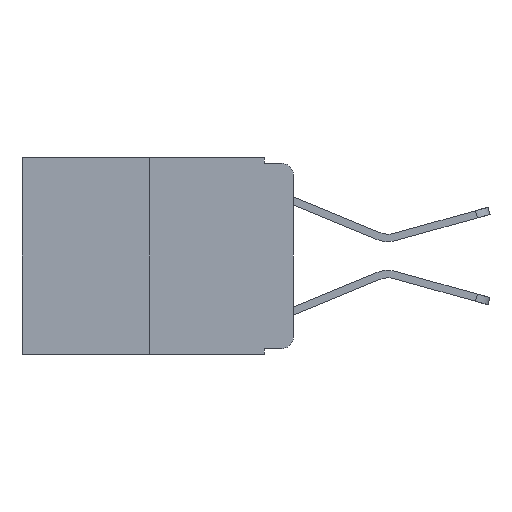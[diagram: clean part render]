
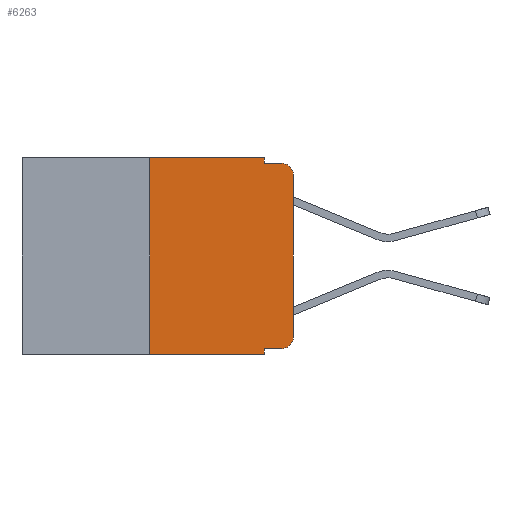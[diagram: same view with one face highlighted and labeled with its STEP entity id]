
A CAD part, left-side view. The second image highlights one B-rep face of the part: STEP entity #6263.
In plain terms, the highlighted planar face has unit normal (-1, 0, 0).
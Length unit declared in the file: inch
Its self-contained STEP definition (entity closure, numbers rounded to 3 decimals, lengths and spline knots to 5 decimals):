
#77 = VECTOR ( 'NONE', #7311, 39.37008 ) ;
#252 = VERTEX_POINT ( 'NONE', #10758 ) ;
#463 = LINE ( 'NONE', #9834, #77 ) ;
#479 = ORIENTED_EDGE ( 'NONE', *, *, #2550, .T. ) ;
#576 = CARTESIAN_POINT ( 'NONE',  ( 0., 0.051, -0.333 ) ) ;
#815 = VECTOR ( 'NONE', #9298, 39.37008 ) ;
#1189 = ORIENTED_EDGE ( 'NONE', *, *, #2565, .F. ) ;
#1667 = DIRECTION ( 'NONE',  ( 0., 0., -1. ) ) ;
#1753 = EDGE_CURVE ( 'NONE', #12235, #2693, #11513, .T. ) ;
#1758 = CARTESIAN_POINT ( 'NONE',  ( 0., 0.051, 0. ) ) ;
#2228 = EDGE_CURVE ( 'NONE', #6107, #11662, #3410, .T. ) ;
#2370 = CARTESIAN_POINT ( 'NONE',  ( 0., 0.02, -0.01 ) ) ;
#2532 = EDGE_CURVE ( 'NONE', #10820, #252, #11505, .T. ) ;
#2550 = EDGE_CURVE ( 'NONE', #252, #9981, #5945, .T. ) ;
#2552 = EDGE_CURVE ( 'NONE', #10318, #9981, #10676, .T. ) ;
#2565 = EDGE_CURVE ( 'NONE', #2693, #10318, #3234, .T. ) ;
#2580 = EDGE_CURVE ( 'NONE', #6107, #12235, #463, .T. ) ;
#2595 = EDGE_CURVE ( 'NONE', #3729, #11662, #2916, .T. ) ;
#2608 = EDGE_CURVE ( 'NONE', #3729, #10895, #10418, .T. ) ;
#2610 = EDGE_CURVE ( 'NONE', #10895, #10820, #5621, .T. ) ;
#2614 = VECTOR ( 'NONE', #9416, 39.37008 ) ;
#2693 = VERTEX_POINT ( 'NONE', #1758 ) ;
#2824 = CARTESIAN_POINT ( 'NONE',  ( 0., 0.25, -0.343 ) ) ;
#2873 = AXIS2_PLACEMENT_3D ( 'NONE', #7110, #12288, #1667 ) ;
#2916 = LINE ( 'NONE', #10233, #7987 ) ;
#3234 = LINE ( 'NONE', #4665, #815 ) ;
#3410 = LINE ( 'NONE', #9201, #10819 ) ;
#3729 = VERTEX_POINT ( 'NONE', #576 ) ;
#3899 = ORIENTED_EDGE ( 'NONE', *, *, #2580, .F. ) ;
#4074 = CARTESIAN_POINT ( 'NONE',  ( 0., 0., 0. ) ) ;
#4325 = DIRECTION ( 'NONE',  ( -1., 0., 0. ) ) ;
#4483 = DIRECTION ( 'NONE',  ( 0., 0., -1. ) ) ;
#4500 = CARTESIAN_POINT ( 'NONE',  ( 0., 0.02, -0.03 ) ) ;
#4665 = CARTESIAN_POINT ( 'NONE',  ( 0., 0.051, 0. ) ) ;
#5621 = CIRCLE ( 'NONE', #6164, 0.02 ) ;
#5795 = DIRECTION ( 'NONE',  ( 0., 0., -1. ) ) ;
#5832 = DIRECTION ( 'NONE',  ( -1., 0., 0. ) ) ;
#5945 = CIRCLE ( 'NONE', #10836, 0.02 ) ;
#5956 = ORIENTED_EDGE ( 'NONE', *, *, #2228, .T. ) ;
#6047 = CARTESIAN_POINT ( 'NONE',  ( 0., 0.051, -0.333 ) ) ;
#6105 = DIRECTION ( 'NONE',  ( 0., 0., 1. ) ) ;
#6107 = VERTEX_POINT ( 'NONE', #2824 ) ;
#6137 = CARTESIAN_POINT ( 'NONE',  ( 0., 0.051, -0.01 ) ) ;
#6164 = AXIS2_PLACEMENT_3D ( 'NONE', #12447, #5832, #5795 ) ;
#6263 = ADVANCED_FACE ( 'NONE', ( #6499 ), #7469, .F. ) ;
#6269 = VECTOR ( 'NONE', #6105, 39.37008 ) ;
#6283 = ORIENTED_EDGE ( 'NONE', *, *, #2552, .F. ) ;
#6499 = FACE_OUTER_BOUND ( 'NONE', #6947, .T. ) ;
#6568 = CARTESIAN_POINT ( 'NONE',  ( 0., 0.25, 0. ) ) ;
#6618 = VECTOR ( 'NONE', #10163, 39.37008 ) ;
#6619 = ORIENTED_EDGE ( 'NONE', *, *, #2608, .T. ) ;
#6749 = CARTESIAN_POINT ( 'NONE',  ( 0., 0.051, -0.01 ) ) ;
#6929 = CARTESIAN_POINT ( 'NONE',  ( 0., 0.051, -0.343 ) ) ;
#6947 = EDGE_LOOP ( 'NONE', ( #8316, #479, #6283, #1189, #8879, #3899, #5956, #9458, #6619, #9181 ) ) ;
#7110 = CARTESIAN_POINT ( 'NONE',  ( 0., 0.473, 0. ) ) ;
#7311 = DIRECTION ( 'NONE',  ( 0., 0., 1. ) ) ;
#7469 = PLANE ( 'NONE',  #2873 ) ;
#7987 = VECTOR ( 'NONE', #9217, 39.37008 ) ;
#8300 = VECTOR ( 'NONE', #9545, 39.37008 ) ;
#8316 = ORIENTED_EDGE ( 'NONE', *, *, #2532, .T. ) ;
#8358 = DIRECTION ( 'NONE',  ( 0., -1., 0. ) ) ;
#8454 = CARTESIAN_POINT ( 'NONE',  ( 0., 0., -0.313 ) ) ;
#8879 = ORIENTED_EDGE ( 'NONE', *, *, #1753, .F. ) ;
#9181 = ORIENTED_EDGE ( 'NONE', *, *, #2610, .T. ) ;
#9201 = CARTESIAN_POINT ( 'NONE',  ( 0., 0.473, -0.343 ) ) ;
#9217 = DIRECTION ( 'NONE',  ( 0., 0., -1. ) ) ;
#9298 = DIRECTION ( 'NONE',  ( 0., 0., -1. ) ) ;
#9416 = DIRECTION ( 'NONE',  ( 0., -1., 0. ) ) ;
#9458 = ORIENTED_EDGE ( 'NONE', *, *, #2595, .F. ) ;
#9545 = DIRECTION ( 'NONE',  ( 0., -1., 0. ) ) ;
#9834 = CARTESIAN_POINT ( 'NONE',  ( 0., 0.25, 0. ) ) ;
#9981 = VERTEX_POINT ( 'NONE', #2370 ) ;
#10163 = DIRECTION ( 'NONE',  ( 0., -1., 0. ) ) ;
#10185 = CARTESIAN_POINT ( 'NONE',  ( 0., 0.473, 0. ) ) ;
#10233 = CARTESIAN_POINT ( 'NONE',  ( 0., 0.051, 0. ) ) ;
#10318 = VERTEX_POINT ( 'NONE', #6749 ) ;
#10418 = LINE ( 'NONE', #6047, #2614 ) ;
#10676 = LINE ( 'NONE', #6137, #8300 ) ;
#10758 = CARTESIAN_POINT ( 'NONE',  ( 0., 0., -0.03 ) ) ;
#10819 = VECTOR ( 'NONE', #8358, 39.37008 ) ;
#10820 = VERTEX_POINT ( 'NONE', #8454 ) ;
#10836 = AXIS2_PLACEMENT_3D ( 'NONE', #4500, #4325, #4483 ) ;
#10895 = VERTEX_POINT ( 'NONE', #11461 ) ;
#11461 = CARTESIAN_POINT ( 'NONE',  ( 0., 0.02, -0.333 ) ) ;
#11505 = LINE ( 'NONE', #4074, #6269 ) ;
#11513 = LINE ( 'NONE', #10185, #6618 ) ;
#11662 = VERTEX_POINT ( 'NONE', #6929 ) ;
#12235 = VERTEX_POINT ( 'NONE', #6568 ) ;
#12288 = DIRECTION ( 'NONE',  ( 1., 0., 0. ) ) ;
#12447 = CARTESIAN_POINT ( 'NONE',  ( 0., 0.02, -0.313 ) ) ;
